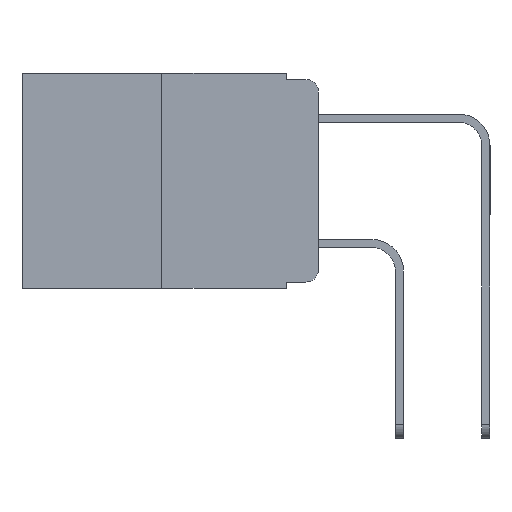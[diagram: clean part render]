
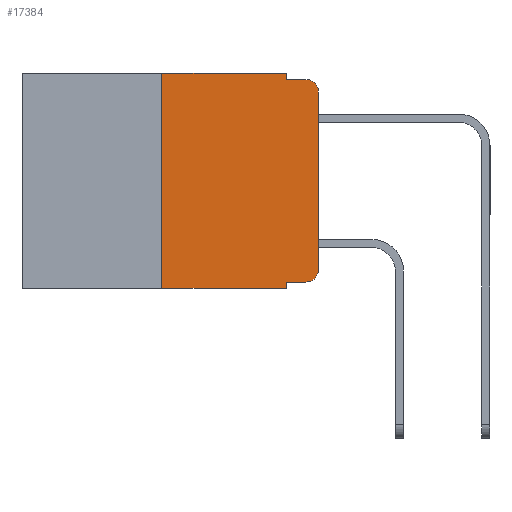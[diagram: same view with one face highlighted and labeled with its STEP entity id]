
A CAD part, left-side view. The second image highlights one B-rep face of the part: STEP entity #17384.
In plain terms, the highlighted planar face has unit normal (-1, 0, 0).
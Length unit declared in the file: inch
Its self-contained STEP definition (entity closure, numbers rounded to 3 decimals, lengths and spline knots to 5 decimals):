
#158 = ORIENTED_EDGE ( 'NONE', *, *, #8962, .F. ) ;
#468 = EDGE_LOOP ( 'NONE', ( #11806, #3719, #8985, #158, #18550, #2324, #2891, #16811, #4005, #5166 ) ) ;
#555 = LINE ( 'NONE', #18497, #17908 ) ;
#808 = DIRECTION ( 'NONE',  ( 0., 0., -1. ) ) ;
#834 = DIRECTION ( 'NONE',  ( -1., 0., 0. ) ) ;
#906 = CARTESIAN_POINT ( 'NONE',  ( 0., 0.02, -0.03 ) ) ;
#943 = LINE ( 'NONE', #11842, #5125 ) ;
#1444 = DIRECTION ( 'NONE',  ( 1., 0., 0. ) ) ;
#1452 = FACE_OUTER_BOUND ( 'NONE', #468, .T. ) ;
#1589 = CARTESIAN_POINT ( 'NONE',  ( 0., 0.25, 0. ) ) ;
#1606 = CARTESIAN_POINT ( 'NONE',  ( 0., 0.051, 0. ) ) ;
#2324 = ORIENTED_EDGE ( 'NONE', *, *, #17461, .F. ) ;
#2353 = VERTEX_POINT ( 'NONE', #5672 ) ;
#2490 = VERTEX_POINT ( 'NONE', #5087 ) ;
#2891 = ORIENTED_EDGE ( 'NONE', *, *, #21287, .T. ) ;
#3147 = VERTEX_POINT ( 'NONE', #17769 ) ;
#3190 = AXIS2_PLACEMENT_3D ( 'NONE', #4197, #15910, #6018 ) ;
#3719 = ORIENTED_EDGE ( 'NONE', *, *, #3910, .T. ) ;
#3910 = EDGE_CURVE ( 'NONE', #16355, #7557, #19682, .T. ) ;
#4005 = ORIENTED_EDGE ( 'NONE', *, *, #16168, .T. ) ;
#4072 = LINE ( 'NONE', #18651, #21072 ) ;
#4197 = CARTESIAN_POINT ( 'NONE',  ( 0., 0.02, -0.313 ) ) ;
#4291 = EDGE_CURVE ( 'NONE', #9726, #5855, #7204, .T. ) ;
#4793 = CARTESIAN_POINT ( 'NONE',  ( 0., 0., 0. ) ) ;
#5085 = AXIS2_PLACEMENT_3D ( 'NONE', #906, #834, #808 ) ;
#5087 = CARTESIAN_POINT ( 'NONE',  ( 0., 0.25, 0. ) ) ;
#5125 = VECTOR ( 'NONE', #15069, 39.37008 ) ;
#5166 = ORIENTED_EDGE ( 'NONE', *, *, #17783, .T. ) ;
#5641 = VECTOR ( 'NONE', #11936, 39.37008 ) ;
#5672 = CARTESIAN_POINT ( 'NONE',  ( 0., 0.02, -0.333 ) ) ;
#5855 = VERTEX_POINT ( 'NONE', #20500 ) ;
#5936 = LINE ( 'NONE', #9150, #10005 ) ;
#6018 = DIRECTION ( 'NONE',  ( 0., 0., -1. ) ) ;
#6097 = CARTESIAN_POINT ( 'NONE',  ( 0., 0.051, -0.01 ) ) ;
#6132 = VECTOR ( 'NONE', #18373, 39.37008 ) ;
#6306 = VECTOR ( 'NONE', #16410, 39.37008 ) ;
#6905 = EDGE_CURVE ( 'NONE', #15771, #16355, #18812, .T. ) ;
#7204 = LINE ( 'NONE', #1606, #6132 ) ;
#7229 = AXIS2_PLACEMENT_3D ( 'NONE', #18150, #1444, #13428 ) ;
#7444 = CARTESIAN_POINT ( 'NONE',  ( 0., 0.02, -0.01 ) ) ;
#7557 = VERTEX_POINT ( 'NONE', #7444 ) ;
#8442 = VERTEX_POINT ( 'NONE', #6097 ) ;
#8962 = EDGE_CURVE ( 'NONE', #18900, #8442, #14776, .T. ) ;
#8968 = EDGE_CURVE ( 'NONE', #2490, #18900, #5936, .T. ) ;
#8985 = ORIENTED_EDGE ( 'NONE', *, *, #13070, .F. ) ;
#9150 = CARTESIAN_POINT ( 'NONE',  ( 0., 0.473, 0. ) ) ;
#9726 = VERTEX_POINT ( 'NONE', #19685 ) ;
#9832 = CARTESIAN_POINT ( 'NONE',  ( 0., 0.051, 0. ) ) ;
#10005 = VECTOR ( 'NONE', #18828, 39.37008 ) ;
#10655 = CARTESIAN_POINT ( 'NONE',  ( 0., 0., -0.03 ) ) ;
#11803 = PLANE ( 'NONE',  #7229 ) ;
#11806 = ORIENTED_EDGE ( 'NONE', *, *, #6905, .T. ) ;
#11842 = CARTESIAN_POINT ( 'NONE',  ( 0., 0.051, -0.333 ) ) ;
#11936 = DIRECTION ( 'NONE',  ( 0., 0., 1. ) ) ;
#12310 = DIRECTION ( 'NONE',  ( 0., -1., 0. ) ) ;
#13070 = EDGE_CURVE ( 'NONE', #8442, #7557, #4072, .T. ) ;
#13428 = DIRECTION ( 'NONE',  ( 0., 0., -1. ) ) ;
#13511 = LINE ( 'NONE', #1589, #5641 ) ;
#13963 = CARTESIAN_POINT ( 'NONE',  ( 0., 0.051, 0. ) ) ;
#14776 = LINE ( 'NONE', #13963, #18507 ) ;
#15069 = DIRECTION ( 'NONE',  ( 0., -1., 0. ) ) ;
#15628 = DIRECTION ( 'NONE',  ( 0., 0., -1. ) ) ;
#15771 = VERTEX_POINT ( 'NONE', #17292 ) ;
#15910 = DIRECTION ( 'NONE',  ( -1., 0., 0. ) ) ;
#16168 = EDGE_CURVE ( 'NONE', #9726, #2353, #943, .T. ) ;
#16355 = VERTEX_POINT ( 'NONE', #10655 ) ;
#16410 = DIRECTION ( 'NONE',  ( 0., 0., 1. ) ) ;
#16811 = ORIENTED_EDGE ( 'NONE', *, *, #4291, .F. ) ;
#16953 = DIRECTION ( 'NONE',  ( 0., -1., 0. ) ) ;
#17292 = CARTESIAN_POINT ( 'NONE',  ( 0., 0., -0.313 ) ) ;
#17384 = ADVANCED_FACE ( 'NONE', ( #1452 ), #11803, .F. ) ;
#17461 = EDGE_CURVE ( 'NONE', #3147, #2490, #13511, .T. ) ;
#17769 = CARTESIAN_POINT ( 'NONE',  ( 0., 0.25, -0.343 ) ) ;
#17783 = EDGE_CURVE ( 'NONE', #2353, #15771, #19700, .T. ) ;
#17908 = VECTOR ( 'NONE', #16953, 39.37008 ) ;
#18150 = CARTESIAN_POINT ( 'NONE',  ( 0., 0.473, 0. ) ) ;
#18373 = DIRECTION ( 'NONE',  ( 0., 0., -1. ) ) ;
#18497 = CARTESIAN_POINT ( 'NONE',  ( 0., 0.473, -0.343 ) ) ;
#18507 = VECTOR ( 'NONE', #15628, 39.37008 ) ;
#18550 = ORIENTED_EDGE ( 'NONE', *, *, #8968, .F. ) ;
#18651 = CARTESIAN_POINT ( 'NONE',  ( 0., 0.051, -0.01 ) ) ;
#18812 = LINE ( 'NONE', #4793, #6306 ) ;
#18828 = DIRECTION ( 'NONE',  ( 0., -1., 0. ) ) ;
#18900 = VERTEX_POINT ( 'NONE', #9832 ) ;
#19682 = CIRCLE ( 'NONE', #5085, 0.02 ) ;
#19685 = CARTESIAN_POINT ( 'NONE',  ( 0., 0.051, -0.333 ) ) ;
#19700 = CIRCLE ( 'NONE', #3190, 0.02 ) ;
#20500 = CARTESIAN_POINT ( 'NONE',  ( 0., 0.051, -0.343 ) ) ;
#21072 = VECTOR ( 'NONE', #12310, 39.37008 ) ;
#21287 = EDGE_CURVE ( 'NONE', #3147, #5855, #555, .T. ) ;
